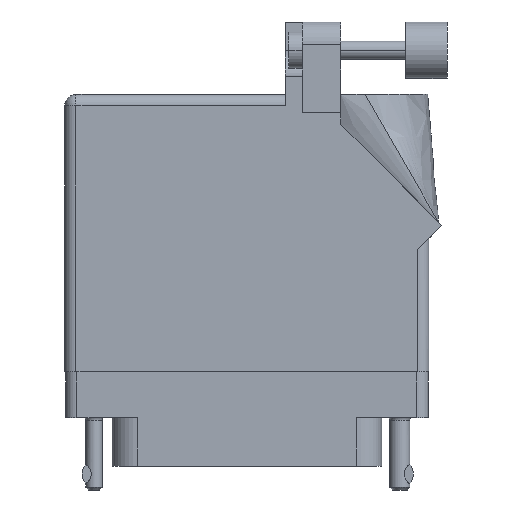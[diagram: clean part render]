
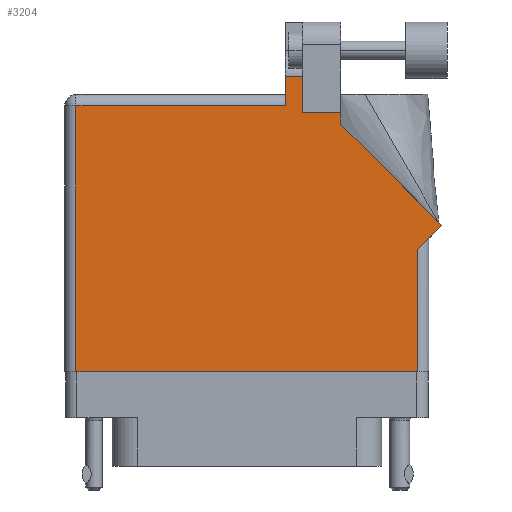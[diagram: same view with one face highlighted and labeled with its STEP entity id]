
A CAD part, front view. The second image highlights one B-rep face of the part: STEP entity #3204.
In plain terms, the highlighted face is planar.
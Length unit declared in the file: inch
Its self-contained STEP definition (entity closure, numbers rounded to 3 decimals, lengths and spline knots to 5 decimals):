
#405 = LINE ( 'NONE', #38829, #14573 ) ;
#1856 = DIRECTION ( 'NONE',  ( -1., 0., 0. ) ) ;
#2357 = VERTEX_POINT ( 'NONE', #45151 ) ;
#2843 = CARTESIAN_POINT ( 'NONE',  ( -1.005, 1.43, 0.455 ) ) ;
#3204 = ADVANCED_FACE ( 'NONE', ( #25675 ), #41015, .F. ) ;
#3400 = ORIENTED_EDGE ( 'NONE', *, *, #48109, .T. ) ;
#4418 = LINE ( 'NONE', #23217, #39788 ) ;
#4932 = EDGE_LOOP ( 'NONE', ( #31431, #5801, #10426, #48120, #7276, #21110, #15487, #39280, #3400, #31637, #14477 ) ) ;
#5029 = VECTOR ( 'NONE', #22799, 39.37008 ) ;
#5801 = ORIENTED_EDGE ( 'NONE', *, *, #34483, .T. ) ;
#7276 = ORIENTED_EDGE ( 'NONE', *, *, #23926, .T. ) ;
#7382 = LINE ( 'NONE', #22686, #48072 ) ;
#7906 = LINE ( 'NONE', #34069, #37798 ) ;
#8414 = EDGE_CURVE ( 'NONE', #46817, #24555, #7382, .T. ) ;
#8468 = CARTESIAN_POINT ( 'NONE',  ( -1.005, 1.368, 0.455 ) ) ;
#10000 = DIRECTION ( 'NONE',  ( 0., 1., 0. ) ) ;
#10426 = ORIENTED_EDGE ( 'NONE', *, *, #25366, .T. ) ;
#10582 = CARTESIAN_POINT ( 'NONE',  ( 0.943, -0.1, 0.455 ) ) ;
#10627 = DIRECTION ( 'NONE',  ( 0., 0., -1. ) ) ;
#11202 = DIRECTION ( 'NONE',  ( 1., 0., 0. ) ) ;
#12695 = VERTEX_POINT ( 'NONE', #45848 ) ;
#12697 = LINE ( 'NONE', #8468, #42171 ) ;
#12779 = CARTESIAN_POINT ( 'NONE',  ( 0.306, 1.33, 0.455 ) ) ;
#12894 = VERTEX_POINT ( 'NONE', #21200 ) ;
#13130 = CARTESIAN_POINT ( 'NONE',  ( 0.63677, 1.5315, 0.455 ) ) ;
#13196 = DIRECTION ( 'NONE',  ( 0., -1., 0. ) ) ;
#13930 = VECTOR ( 'NONE', #25076, 39.37008 ) ;
#13984 = DIRECTION ( 'NONE',  ( 0., 1., 0. ) ) ;
#14477 = ORIENTED_EDGE ( 'NONE', *, *, #49471, .T. ) ;
#14573 = VECTOR ( 'NONE', #41587, 39.37008 ) ;
#14782 = LINE ( 'NONE', #42365, #5029 ) ;
#15487 = ORIENTED_EDGE ( 'NONE', *, *, #22190, .T. ) ;
#16771 = VERTEX_POINT ( 'NONE', #10582 ) ;
#17987 = LINE ( 'NONE', #32843, #29132 ) ;
#19038 = EDGE_CURVE ( 'NONE', #21587, #24720, #29553, .T. ) ;
#20438 = CARTESIAN_POINT ( 'NONE',  ( 0.212, 1.5315, 0.455 ) ) ;
#20986 = DIRECTION ( 'NONE',  ( -1., 0., 0. ) ) ;
#21110 = ORIENTED_EDGE ( 'NONE', *, *, #34715, .T. ) ;
#21200 = CARTESIAN_POINT ( 'NONE',  ( -0.943, 1.368, 0.455 ) ) ;
#21587 = VERTEX_POINT ( 'NONE', #12779 ) ;
#21829 = EDGE_CURVE ( 'NONE', #12695, #27554, #14782, .T. ) ;
#22190 = EDGE_CURVE ( 'NONE', #16771, #46817, #17987, .T. ) ;
#22602 = CARTESIAN_POINT ( 'NONE',  ( 0.212, 1.368, 0.455 ) ) ;
#22686 = CARTESIAN_POINT ( 'NONE',  ( 1.005, 0.637, 0.455 ) ) ;
#22797 = CARTESIAN_POINT ( 'NONE',  ( 0.519, 1.33, 0.455 ) ) ;
#22799 = DIRECTION ( 'NONE',  ( 0., 1., 0. ) ) ;
#23217 = CARTESIAN_POINT ( 'NONE',  ( -1.005, -0.1, 0.455 ) ) ;
#23926 = EDGE_CURVE ( 'NONE', #12894, #2357, #25228, .T. ) ;
#24555 = VERTEX_POINT ( 'NONE', #47934 ) ;
#24720 = VERTEX_POINT ( 'NONE', #30997 ) ;
#25076 = DIRECTION ( 'NONE',  ( 0., -1., 0. ) ) ;
#25228 = LINE ( 'NONE', #40569, #37085 ) ;
#25366 = EDGE_CURVE ( 'NONE', #46055, #37696, #37161, .T. ) ;
#25675 = FACE_OUTER_BOUND ( 'NONE', #4932, .T. ) ;
#25943 = DIRECTION ( 'NONE',  ( -1., 0., 0. ) ) ;
#27554 = VERTEX_POINT ( 'NONE', #22797 ) ;
#28466 = LINE ( 'NONE', #13130, #30960 ) ;
#29132 = VECTOR ( 'NONE', #13984, 39.37008 ) ;
#29553 = LINE ( 'NONE', #36386, #41729 ) ;
#30960 = VECTOR ( 'NONE', #1856, 39.37008 ) ;
#30997 = CARTESIAN_POINT ( 'NONE',  ( 0.306, 1.5315, 0.455 ) ) ;
#31431 = ORIENTED_EDGE ( 'NONE', *, *, #19038, .T. ) ;
#31637 = ORIENTED_EDGE ( 'NONE', *, *, #21829, .T. ) ;
#32843 = CARTESIAN_POINT ( 'NONE',  ( 0.943, 0.637, 0.455 ) ) ;
#34069 = CARTESIAN_POINT ( 'NONE',  ( 1.07571, 0.70771, 0.455 ) ) ;
#34483 = EDGE_CURVE ( 'NONE', #24720, #46055, #28466, .T. ) ;
#34715 = EDGE_CURVE ( 'NONE', #2357, #16771, #4418, .T. ) ;
#35280 = CARTESIAN_POINT ( 'NONE',  ( 0.943, 0.575, 0.455 ) ) ;
#36386 = CARTESIAN_POINT ( 'NONE',  ( 0.306, 1.33, 0.455 ) ) ;
#36535 = EDGE_CURVE ( 'NONE', #37696, #12894, #12697, .T. ) ;
#37085 = VECTOR ( 'NONE', #13196, 39.37008 ) ;
#37161 = LINE ( 'NONE', #40655, #13930 ) ;
#37696 = VERTEX_POINT ( 'NONE', #22602 ) ;
#37798 = VECTOR ( 'NONE', #42299, 39.37008 ) ;
#38506 = DIRECTION ( 'NONE',  ( 0.707, 0.707, 0. ) ) ;
#38829 = CARTESIAN_POINT ( 'NONE',  ( 0.519, 1.33, 0.455 ) ) ;
#39280 = ORIENTED_EDGE ( 'NONE', *, *, #8414, .T. ) ;
#39788 = VECTOR ( 'NONE', #11202, 39.37008 ) ;
#40569 = CARTESIAN_POINT ( 'NONE',  ( -0.943, -0.1, 0.455 ) ) ;
#40655 = CARTESIAN_POINT ( 'NONE',  ( 0.212, 1.43, 0.455 ) ) ;
#41015 = PLANE ( 'NONE',  #44978 ) ;
#41587 = DIRECTION ( 'NONE',  ( -1., 0., 0. ) ) ;
#41729 = VECTOR ( 'NONE', #10000, 39.37008 ) ;
#42171 = VECTOR ( 'NONE', #20986, 39.37008 ) ;
#42299 = DIRECTION ( 'NONE',  ( -0.707, 0.707, 0. ) ) ;
#42365 = CARTESIAN_POINT ( 'NONE',  ( 0.519, 1.26442, 0.455 ) ) ;
#44978 = AXIS2_PLACEMENT_3D ( 'NONE', #2843, #10627, #25943 ) ;
#45151 = CARTESIAN_POINT ( 'NONE',  ( -0.943, -0.1, 0.455 ) ) ;
#45848 = CARTESIAN_POINT ( 'NONE',  ( 0.519, 1.26442, 0.455 ) ) ;
#46055 = VERTEX_POINT ( 'NONE', #20438 ) ;
#46817 = VERTEX_POINT ( 'NONE', #35280 ) ;
#47934 = CARTESIAN_POINT ( 'NONE',  ( 1.07571, 0.70771, 0.455 ) ) ;
#48072 = VECTOR ( 'NONE', #38506, 39.37008 ) ;
#48109 = EDGE_CURVE ( 'NONE', #24555, #12695, #7906, .T. ) ;
#48120 = ORIENTED_EDGE ( 'NONE', *, *, #36535, .T. ) ;
#49471 = EDGE_CURVE ( 'NONE', #27554, #21587, #405, .T. ) ;
